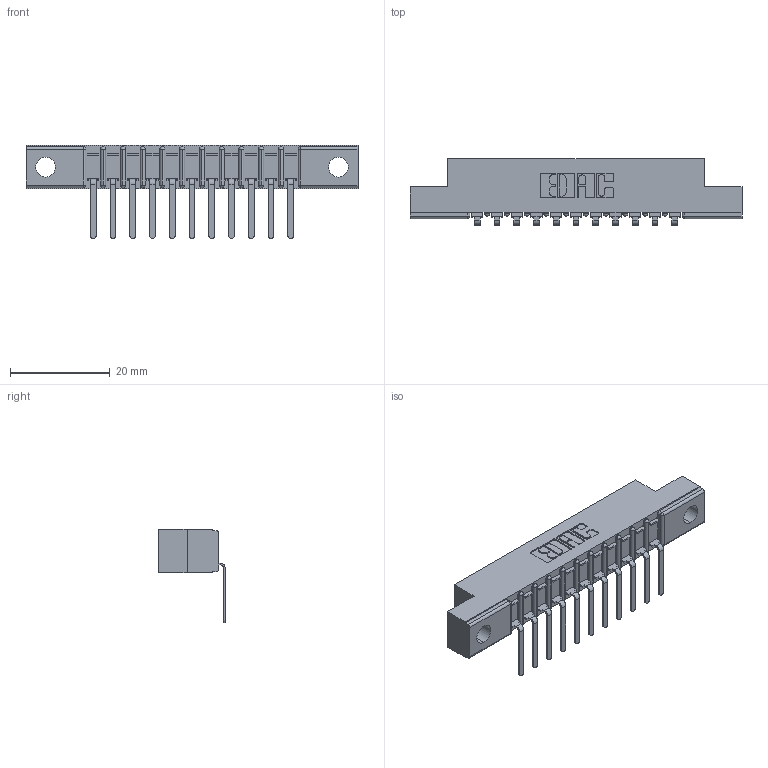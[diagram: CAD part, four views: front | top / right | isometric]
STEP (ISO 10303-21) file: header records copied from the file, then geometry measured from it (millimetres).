
FILE_DESCRIPTION (( 'STEP AP203' ), '1' );
FILE_NAME ('357-011-557-104.STEP', '2019-09-16T19:01:41', ( '' ), ( '' ), 'SwSTEP 2.0', 'SolidWorks 2016', '' );
FILE_SCHEMA (( 'CONFIG_CONTROL_DESIGN' ));
Length unit declared in the file: inch
Products named in the file (3): 307-290-002_557; 357-011-557-104; 307 Part_.156 Dia Mounting Holes
Assembly tree (12 placements, depth 2):
  357-011-557-104
    307 Part_.156 Dia Mounting Holes
    307-290-002_557  x11
Bounding box: 66.6 x 13.32 x 18.67 mm (x, y, z)
Volume: 4314.7 mm3; surface area: 7308.2 mm2
Topology: 12 solids, 12 shells, 1002 faces, 3043 edges, 1994 vertices
Faces by surface type: plane 601, cylinder 377, sphere 24
Entity records: 14524 total; most frequent: CARTESIAN_POINT 2450, ORIENTED_EDGE 2438, DIRECTION 2387, EDGE_CURVE 1219, LINE 925, VECTOR 925, VERTEX_POINT 794, AXIS2_PLACEMENT_3D 731
